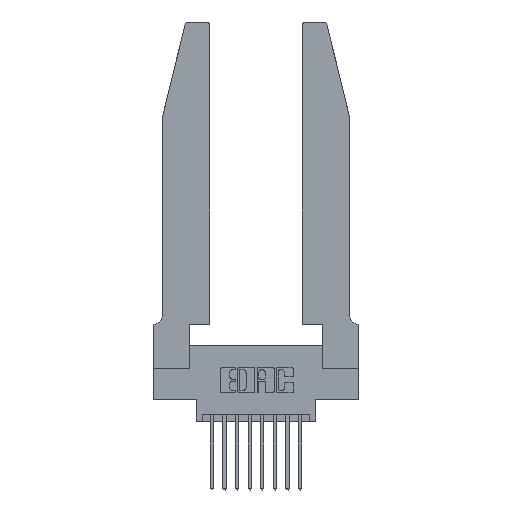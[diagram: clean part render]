
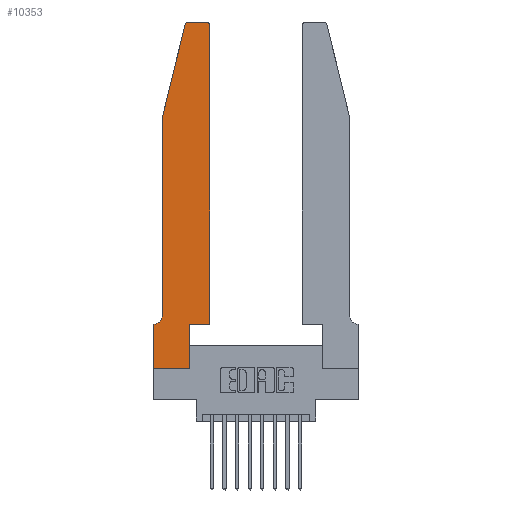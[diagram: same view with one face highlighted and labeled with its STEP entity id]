
A CAD part, top view. The second image highlights one B-rep face of the part: STEP entity #10353.
In plain terms, the highlighted planar face has unit normal (0, 0, 1).
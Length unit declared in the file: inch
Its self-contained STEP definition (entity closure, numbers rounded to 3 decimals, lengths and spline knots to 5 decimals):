
#113 = DIRECTION ( 'NONE',  ( 1., 0., 0. ) ) ;
#129 = ORIENTED_EDGE ( 'NONE', *, *, #2487, .T. ) ;
#144 = CARTESIAN_POINT ( 'NONE',  ( 0., 0.35, 0.37 ) ) ;
#207 = VECTOR ( 'NONE', #15446, 39.37008 ) ;
#403 = ORIENTED_EDGE ( 'NONE', *, *, #8297, .T. ) ;
#468 = EDGE_LOOP ( 'NONE', ( #14735, #13587, #4638, #129, #2257, #12565, #403, #11988, #2374, #4673, #10337, #9454 ) ) ;
#1234 = CARTESIAN_POINT ( 'NONE',  ( 0., 0., 0.37 ) ) ;
#1362 = CARTESIAN_POINT ( 'NONE',  ( 0.0755, 0.35, 0.37 ) ) ;
#1416 = VECTOR ( 'NONE', #6034, 39.37008 ) ;
#1538 = DIRECTION ( 'NONE',  ( -1., 0., 0. ) ) ;
#1551 = EDGE_CURVE ( 'NONE', #1589, #6181, #1804, .T. ) ;
#1573 = EDGE_CURVE ( 'NONE', #7235, #12229, #4237, .T. ) ;
#1585 = VERTEX_POINT ( 'NONE', #15360 ) ;
#1589 = VERTEX_POINT ( 'NONE', #15342 ) ;
#1804 = LINE ( 'NONE', #4889, #14710 ) ;
#2190 = EDGE_CURVE ( 'NONE', #12229, #10137, #15250, .T. ) ;
#2237 = CARTESIAN_POINT ( 'NONE',  ( 0.4505, 0.35, 0.37 ) ) ;
#2257 = ORIENTED_EDGE ( 'NONE', *, *, #2572, .T. ) ;
#2309 = LINE ( 'NONE', #1362, #8398 ) ;
#2359 = EDGE_CURVE ( 'NONE', #12622, #7235, #10161, .T. ) ;
#2374 = ORIENTED_EDGE ( 'NONE', *, *, #2359, .T. ) ;
#2431 = AXIS2_PLACEMENT_3D ( 'NONE', #8400, #8370, #8353 ) ;
#2487 = EDGE_CURVE ( 'NONE', #4167, #15253, #5768, .T. ) ;
#2572 = EDGE_CURVE ( 'NONE', #15253, #1585, #12773, .T. ) ;
#2780 = LINE ( 'NONE', #1234, #15312 ) ;
#2989 = CARTESIAN_POINT ( 'NONE',  ( 0.284, 2.75, 0.37 ) ) ;
#3238 = DIRECTION ( 'NONE',  ( 0., -1., 0. ) ) ;
#3252 = EDGE_CURVE ( 'NONE', #6181, #10708, #10134, .T. ) ;
#3434 = LINE ( 'NONE', #10556, #13507 ) ;
#3442 = CIRCLE ( 'NONE', #14806, 0.03 ) ;
#3463 = CARTESIAN_POINT ( 'NONE',  ( 0.0755, 0.42, 0.37 ) ) ;
#3667 = EDGE_CURVE ( 'NONE', #10708, #4167, #11245, .T. ) ;
#4056 = EDGE_CURVE ( 'NONE', #10137, #1589, #3442, .T. ) ;
#4167 = VERTEX_POINT ( 'NONE', #7437 ) ;
#4193 = CARTESIAN_POINT ( 'NONE',  ( 0.4505, 0.35, 0.37 ) ) ;
#4237 = LINE ( 'NONE', #6747, #1416 ) ;
#4470 = CARTESIAN_POINT ( 'NONE',  ( 0.2865, 0.35, 0.37 ) ) ;
#4607 = VECTOR ( 'NONE', #9421, 39.37008 ) ;
#4638 = ORIENTED_EDGE ( 'NONE', *, *, #3667, .T. ) ;
#4673 = ORIENTED_EDGE ( 'NONE', *, *, #1573, .T. ) ;
#4828 = EDGE_CURVE ( 'NONE', #1585, #10878, #2309, .T. ) ;
#4889 = CARTESIAN_POINT ( 'NONE',  ( 0.2605, 2.75, 0.37 ) ) ;
#4896 = DIRECTION ( 'NONE',  ( 1., 0., 0. ) ) ;
#5101 = DIRECTION ( 'NONE',  ( 0., 0., -1. ) ) ;
#5443 = AXIS2_PLACEMENT_3D ( 'NONE', #10359, #5101, #11437 ) ;
#5768 = LINE ( 'NONE', #7949, #4607 ) ;
#6034 = DIRECTION ( 'NONE',  ( 1., 0., 0. ) ) ;
#6181 = VERTEX_POINT ( 'NONE', #2989 ) ;
#6229 = CARTESIAN_POINT ( 'NONE',  ( 0., 0.35, 0.37 ) ) ;
#6747 = CARTESIAN_POINT ( 'NONE',  ( 0.4505, 0.35, 0.37 ) ) ;
#7235 = VERTEX_POINT ( 'NONE', #4470 ) ;
#7305 = DIRECTION ( 'NONE',  ( -1., 0., 0. ) ) ;
#7437 = CARTESIAN_POINT ( 'NONE',  ( 0.0755, 2., 0.37 ) ) ;
#7448 = DIRECTION ( 'NONE',  ( 0., 0., 1. ) ) ;
#7461 = EDGE_CURVE ( 'NONE', #8427, #12622, #2780, .T. ) ;
#7949 = CARTESIAN_POINT ( 'NONE',  ( 0.0755, 2., 0.37 ) ) ;
#8297 = EDGE_CURVE ( 'NONE', #10878, #8427, #3434, .T. ) ;
#8348 = DIRECTION ( 'NONE',  ( 1., 0., 0. ) ) ;
#8353 = DIRECTION ( 'NONE',  ( 1., 0., 0. ) ) ;
#8370 = DIRECTION ( 'NONE',  ( 0., 0., 1. ) ) ;
#8398 = VECTOR ( 'NONE', #1538, 39.37008 ) ;
#8399 = DIRECTION ( 'NONE',  ( 0., 0., 1. ) ) ;
#8400 = CARTESIAN_POINT ( 'NONE',  ( 0.284, 2.72, 0.37 ) ) ;
#8414 = CARTESIAN_POINT ( 'NONE',  ( 0.4205, 2.72, 0.37 ) ) ;
#8427 = VERTEX_POINT ( 'NONE', #14380 ) ;
#8540 = FACE_OUTER_BOUND ( 'NONE', #468, .T. ) ;
#9421 = DIRECTION ( 'NONE',  ( 0., -1., 0. ) ) ;
#9454 = ORIENTED_EDGE ( 'NONE', *, *, #4056, .T. ) ;
#9788 = VECTOR ( 'NONE', #15048, 39.37008 ) ;
#10134 = CIRCLE ( 'NONE', #2431, 0.03 ) ;
#10137 = VERTEX_POINT ( 'NONE', #13011 ) ;
#10161 = LINE ( 'NONE', #15066, #9788 ) ;
#10337 = ORIENTED_EDGE ( 'NONE', *, *, #2190, .T. ) ;
#10353 = ADVANCED_FACE ( 'NONE', ( #8540 ), #13487, .T. ) ;
#10359 = CARTESIAN_POINT ( 'NONE',  ( 0.0055, 0.42, 0.37 ) ) ;
#10556 = CARTESIAN_POINT ( 'NONE',  ( 0., 0., 0.37 ) ) ;
#10708 = VERTEX_POINT ( 'NONE', #11732 ) ;
#10878 = VERTEX_POINT ( 'NONE', #144 ) ;
#11245 = LINE ( 'NONE', #14029, #11625 ) ;
#11437 = DIRECTION ( 'NONE',  ( -1., 0., 0. ) ) ;
#11625 = VECTOR ( 'NONE', #14265, 39.37008 ) ;
#11680 = AXIS2_PLACEMENT_3D ( 'NONE', #6229, #7448, #113 ) ;
#11732 = CARTESIAN_POINT ( 'NONE',  ( 0.25487, 2.72718, 0.37 ) ) ;
#11988 = ORIENTED_EDGE ( 'NONE', *, *, #7461, .T. ) ;
#12229 = VERTEX_POINT ( 'NONE', #2237 ) ;
#12565 = ORIENTED_EDGE ( 'NONE', *, *, #4828, .T. ) ;
#12622 = VERTEX_POINT ( 'NONE', #15302 ) ;
#12773 = CIRCLE ( 'NONE', #5443, 0.07 ) ;
#13011 = CARTESIAN_POINT ( 'NONE',  ( 0.4505, 2.72, 0.37 ) ) ;
#13487 = PLANE ( 'NONE',  #11680 ) ;
#13507 = VECTOR ( 'NONE', #3238, 39.37008 ) ;
#13587 = ORIENTED_EDGE ( 'NONE', *, *, #3252, .T. ) ;
#14029 = CARTESIAN_POINT ( 'NONE',  ( 0.0755, 2., 0.37 ) ) ;
#14265 = DIRECTION ( 'NONE',  ( -0.239, -0.971, 0. ) ) ;
#14380 = CARTESIAN_POINT ( 'NONE',  ( 0., 0., 0.37 ) ) ;
#14710 = VECTOR ( 'NONE', #7305, 39.37008 ) ;
#14735 = ORIENTED_EDGE ( 'NONE', *, *, #1551, .T. ) ;
#14806 = AXIS2_PLACEMENT_3D ( 'NONE', #8414, #8399, #8348 ) ;
#15048 = DIRECTION ( 'NONE',  ( 0., 1., 0. ) ) ;
#15066 = CARTESIAN_POINT ( 'NONE',  ( 0.2865, 0.35, 0.37 ) ) ;
#15250 = LINE ( 'NONE', #4193, #207 ) ;
#15253 = VERTEX_POINT ( 'NONE', #3463 ) ;
#15302 = CARTESIAN_POINT ( 'NONE',  ( 0.2865, 0., 0.37 ) ) ;
#15312 = VECTOR ( 'NONE', #4896, 39.37008 ) ;
#15342 = CARTESIAN_POINT ( 'NONE',  ( 0.4205, 2.75, 0.37 ) ) ;
#15360 = CARTESIAN_POINT ( 'NONE',  ( 0.0055, 0.35, 0.37 ) ) ;
#15446 = DIRECTION ( 'NONE',  ( 0., 1., 0. ) ) ;
